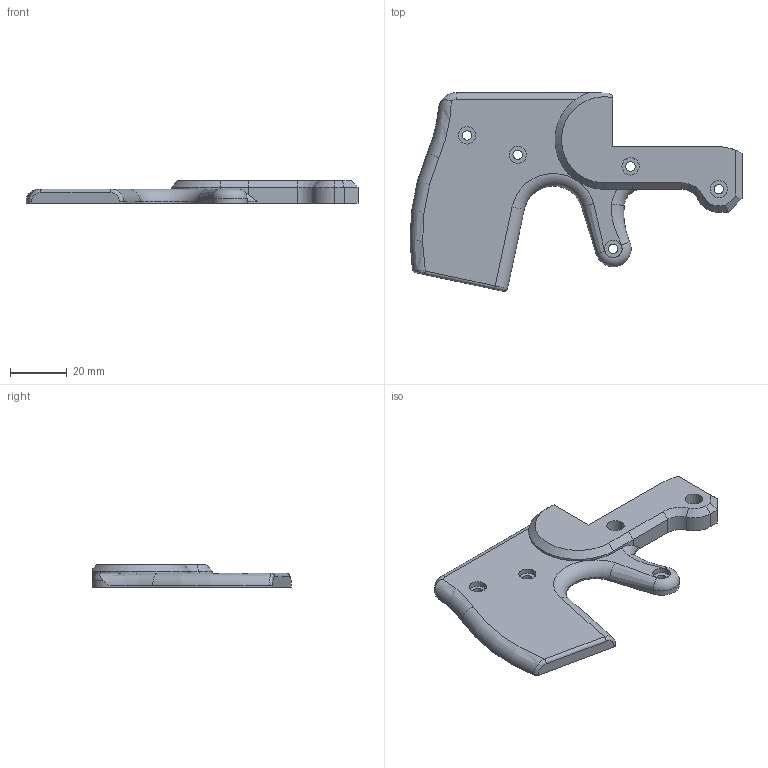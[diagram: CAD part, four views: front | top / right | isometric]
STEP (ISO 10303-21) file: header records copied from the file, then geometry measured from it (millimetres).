
FILE_DESCRIPTION(/* description */ ('STEP AP242','CAx-IF Rec.Pracs.---Representation and Presentation of Product Manufacturing Information (PMI)---4.0---2014-10-13','CAx-IF Rec.Pracs.---3D Tessellated Geometry---0.4---2014-09-14','2;1'),/* implementation_level */ '2;1');
FILE_NAME(/* name */ '61f05f684799ad2097f8dfdd',/* time_stamp */ '2022-01-25T20:36:57+00:00',/* author */ (''),/* organization */ (''),/* preprocessor_version */ 'ST-DEVELOPER v18.101',/* originating_system */ ' ',/* authorisation */ ' ');
FILE_SCHEMA (('AP242_MANAGED_MODEL_BASED_3D_ENGINEERING_MIM_LF { 1 0 10303 442 1 1 4 }'));
Length unit declared in the file: metre
Products named in the file (1): right side frame
Bounding box: 117.49 x 70.33 x 8 mm (x, y, z)
Volume: 25023.9 mm3; surface area: 11825.2 mm2
Topology: 1 solids, 1 shells, 88 faces, 216 edges, 136 vertices
Faces by surface type: plane 40, cylinder 28, cone 9, torus 7, bspline 4
Full cylindrical faces by diameter (mm): 3.302 x5, 6.096 x5
Entity records: 2668 total; most frequent: CARTESIAN_POINT 610, DIRECTION 423, ORIENTED_EDGE 402, EDGE_CURVE 201, AXIS2_PLACEMENT_3D 161, VERTEX_POINT 136, EDGE_LOOP 119, FACE_BOUND 119
